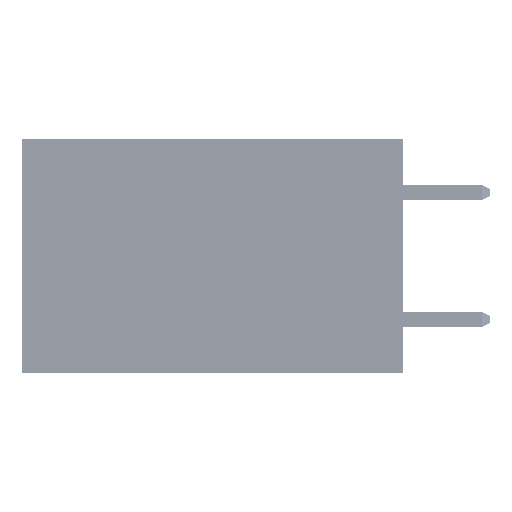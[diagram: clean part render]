
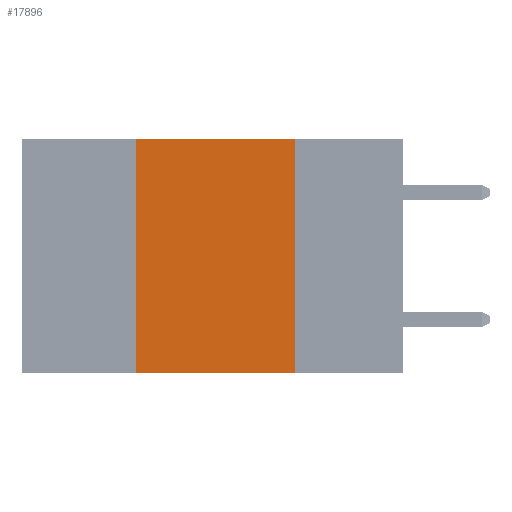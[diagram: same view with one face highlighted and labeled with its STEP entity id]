
A CAD part, left-side view. The second image highlights one B-rep face of the part: STEP entity #17896.
In plain terms, the highlighted planar face has unit normal (-1, 0, 0).
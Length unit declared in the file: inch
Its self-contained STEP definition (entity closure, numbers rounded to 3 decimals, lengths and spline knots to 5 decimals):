
#91 = DIRECTION ( 'NONE',  ( 0., 0., -1. ) ) ;
#1172 = DIRECTION ( 'NONE',  ( 0., 0., 1. ) ) ;
#1661 = LINE ( 'NONE', #13163, #6924 ) ;
#4053 = AXIS2_PLACEMENT_3D ( 'NONE', #11001, #31450, #23812 ) ;
#5226 = ORIENTED_EDGE ( 'NONE', *, *, #31537, .F. ) ;
#6924 = VECTOR ( 'NONE', #45144, 39.37008 ) ;
#10206 = ORIENTED_EDGE ( 'NONE', *, *, #43380, .T. ) ;
#11001 = CARTESIAN_POINT ( 'NONE',  ( 0., 0.6, 0. ) ) ;
#12378 = CARTESIAN_POINT ( 'NONE',  ( 0., 0.17, 0. ) ) ;
#13163 = CARTESIAN_POINT ( 'NONE',  ( 0., 0.6, 0. ) ) ;
#13345 = EDGE_CURVE ( 'NONE', #13524, #28036, #1661, .T. ) ;
#13524 = VERTEX_POINT ( 'NONE', #28593 ) ;
#15602 = CARTESIAN_POINT ( 'NONE',  ( 0., 0.17, -0.37 ) ) ;
#16516 = LINE ( 'NONE', #36430, #20876 ) ;
#17896 = ADVANCED_FACE ( 'NONE', ( #29429 ), #39802, .F. ) ;
#20663 = ORIENTED_EDGE ( 'NONE', *, *, #27594, .F. ) ;
#20876 = VECTOR ( 'NONE', #49000, 39.37008 ) ;
#23054 = EDGE_LOOP ( 'NONE', ( #20663, #33520, #5226, #10206 ) ) ;
#23812 = DIRECTION ( 'NONE',  ( 0., 0., -1. ) ) ;
#27594 = EDGE_CURVE ( 'NONE', #28036, #41050, #28872, .T. ) ;
#28036 = VERTEX_POINT ( 'NONE', #51135 ) ;
#28593 = CARTESIAN_POINT ( 'NONE',  ( 0., 0.42, 0. ) ) ;
#28872 = LINE ( 'NONE', #12378, #47173 ) ;
#29429 = FACE_OUTER_BOUND ( 'NONE', #23054, .T. ) ;
#31450 = DIRECTION ( 'NONE',  ( 1., 0., 0. ) ) ;
#31537 = EDGE_CURVE ( 'NONE', #51069, #13524, #44420, .T. ) ;
#33520 = ORIENTED_EDGE ( 'NONE', *, *, #13345, .F. ) ;
#36430 = CARTESIAN_POINT ( 'NONE',  ( 0., 0.6, -0.37 ) ) ;
#37056 = CARTESIAN_POINT ( 'NONE',  ( 0., 0.42, 0. ) ) ;
#39802 = PLANE ( 'NONE',  #4053 ) ;
#41050 = VERTEX_POINT ( 'NONE', #15602 ) ;
#43380 = EDGE_CURVE ( 'NONE', #51069, #41050, #16516, .T. ) ;
#44420 = LINE ( 'NONE', #37056, #47946 ) ;
#45144 = DIRECTION ( 'NONE',  ( 0., -1., 0. ) ) ;
#47173 = VECTOR ( 'NONE', #91, 39.37008 ) ;
#47946 = VECTOR ( 'NONE', #1172, 39.37008 ) ;
#48909 = CARTESIAN_POINT ( 'NONE',  ( 0., 0.42, -0.37 ) ) ;
#49000 = DIRECTION ( 'NONE',  ( 0., -1., 0. ) ) ;
#51069 = VERTEX_POINT ( 'NONE', #48909 ) ;
#51135 = CARTESIAN_POINT ( 'NONE',  ( 0., 0.17, 0. ) ) ;
